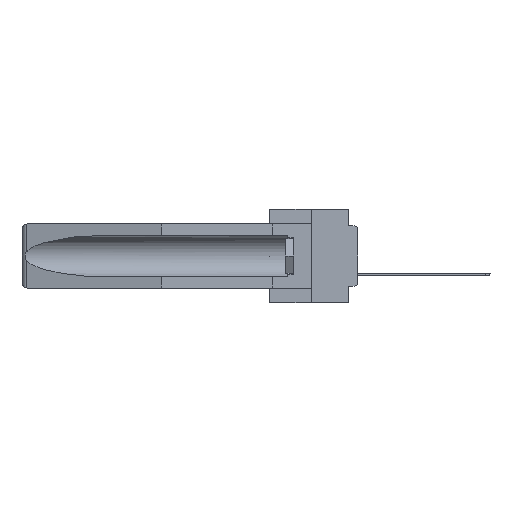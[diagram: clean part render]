
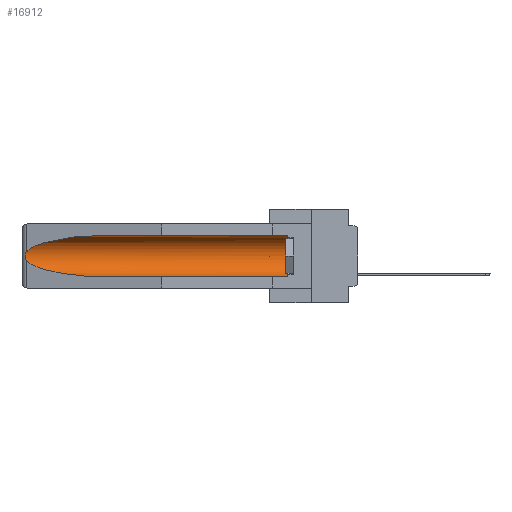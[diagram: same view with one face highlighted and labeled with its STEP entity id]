
A CAD part, left-side view. The second image highlights one B-rep face of the part: STEP entity #16912.
In plain terms, the highlighted cylindrical face has radius 2.857 mm (diameter 5.715 mm), a partial arc.
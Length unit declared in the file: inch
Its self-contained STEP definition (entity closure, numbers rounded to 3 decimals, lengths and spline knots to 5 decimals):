
#337 = ORIENTED_EDGE ( 'NONE', *, *, #30205, .T. ) ;
#547 = FACE_OUTER_BOUND ( 'NONE', #31885, .T. ) ;
#1500 = CARTESIAN_POINT ( 'NONE',  ( 0.155, 0.126, -0.059 ) ) ;
#3882 = CARTESIAN_POINT ( 'NONE',  ( 0.26654, 1.53092, -0.15636 ) ) ;
#4291 = DIRECTION ( 'NONE',  ( 0., 1., 0. ) ) ;
#4937 = CARTESIAN_POINT ( 'NONE',  ( 0.155, -0.30754, -0.284 ) ) ;
#4938 = CARTESIAN_POINT ( 'NONE',  ( 0.155, 0.126, -0.1715 ) ) ;
#5771 = ORIENTED_EDGE ( 'NONE', *, *, #23703, .T. ) ;
#5797 = CARTESIAN_POINT ( 'NONE',  ( 0.21114, 1.30732, -0.059 ) ) ;
#6588 = CARTESIAN_POINT ( 'NONE',  ( 0.2675, 1.53308, -0.16763 ) ) ;
#8005 = VECTOR ( 'NONE', #28163, 39.37008 ) ;
#9463 = CARTESIAN_POINT ( 'NONE',  ( 0.2673, 1.5327, -0.16383 ) ) ;
#11880 = VERTEX_POINT ( 'NONE', #34142 ) ;
#12299 = CARTESIAN_POINT ( 'NONE',  ( 0.26537, 1.52718, -0.19328 ) ) ;
#12626 = LINE ( 'NONE', #4937, #8005 ) ;
#13645 = EDGE_CURVE ( 'NONE', #19716, #15013, #28660, .T. ) ;
#15013 = VERTEX_POINT ( 'NONE', #1500 ) ;
#15052 = ORIENTED_EDGE ( 'NONE', *, *, #20947, .F. ) ;
#15313 = CARTESIAN_POINT ( 'NONE',  ( 0.26597, 1.52961, -0.15275 ) ) ;
#15437 = CARTESIAN_POINT ( 'NONE',  ( 0.26537, 1.52718, -0.14972 ) ) ;
#15881 = CARTESIAN_POINT ( 'NONE',  ( 0.155, 1.07973, -0.059 ) ) ;
#16110 = CARTESIAN_POINT ( 'NONE',  ( 0.155, 0.126, -0.284 ) ) ;
#16495 = EDGE_CURVE ( 'NONE', #33585, #11880, #25370, .T. ) ;
#16912 = ADVANCED_FACE ( 'NONE', ( #547 ), #29380, .F. ) ;
#17400 = AXIS2_PLACEMENT_3D ( 'NONE', #4938, #25728, #37109 ) ;
#18661 = VERTEX_POINT ( 'NONE', #15881 ) ;
#18702 = CARTESIAN_POINT ( 'NONE',  ( 0.2673, 1.53269, -0.17917 ) ) ;
#19716 = VERTEX_POINT ( 'NONE', #16110 ) ;
#19868 = VECTOR ( 'NONE', #36166, 39.37008 ) ;
#20947 = EDGE_CURVE ( 'NONE', #19716, #23461, #12626, .T. ) ;
#22283 = CARTESIAN_POINT ( 'NONE',  ( 0.26537, 1.52718, -0.19328 ) ) ;
#22525 =( BOUNDED_CURVE ( )  B_SPLINE_CURVE ( 3, ( #34262, #5797, #32689, #24079 ),
 .UNSPECIFIED., .F., .F. ) 
 B_SPLINE_CURVE_WITH_KNOTS ( ( 4, 4 ),
 ( 4.71239, 6.08839 ),
 .UNSPECIFIED. ) 
 CURVE ( )  GEOMETRIC_REPRESENTATION_ITEM ( )  RATIONAL_B_SPLINE_CURVE ( ( 1., 0.848, 0.848, 1. ) ) 
 REPRESENTATION_ITEM ( '' )  );
#23461 = VERTEX_POINT ( 'NONE', #33996 ) ;
#23484 = ORIENTED_EDGE ( 'NONE', *, *, #23903, .T. ) ;
#23703 = EDGE_CURVE ( 'NONE', #11880, #23461, #29368, .T. ) ;
#23903 = EDGE_CURVE ( 'NONE', #15013, #18661, #27678, .T. ) ;
#24079 = CARTESIAN_POINT ( 'NONE',  ( 0.26537, 1.52718, -0.14972 ) ) ;
#24775 = CARTESIAN_POINT ( 'NONE',  ( 0.155, -0.30754, -0.059 ) ) ;
#24996 = CARTESIAN_POINT ( 'NONE',  ( 0.155, 1.07973, -0.284 ) ) ;
#25285 = CARTESIAN_POINT ( 'NONE',  ( 0.25451, 1.48313, -0.24835 ) ) ;
#25370 = B_SPLINE_CURVE_WITH_KNOTS ( 'NONE', 3,
 ( #15437, #15313, #3882, #9463, #6588, #30485, #18702, #33081, #36181, #12299 ),
 .UNSPECIFIED., .F., .F.,
 ( 4, 2, 2, 2, 4 ),
 ( 0., 0.00029, 0.00058, 0.00087, 0.00117 ),
 .UNSPECIFIED. ) ;
#25728 = DIRECTION ( 'NONE',  ( 0., -1., 0. ) ) ;
#26277 = ORIENTED_EDGE ( 'NONE', *, *, #16495, .T. ) ;
#27678 = LINE ( 'NONE', #24775, #19868 ) ;
#27808 = CARTESIAN_POINT ( 'NONE',  ( 0.26537, 1.52718, -0.14972 ) ) ;
#27814 = ORIENTED_EDGE ( 'NONE', *, *, #13645, .T. ) ;
#28163 = DIRECTION ( 'NONE',  ( 0., 1., 0. ) ) ;
#28347 = CARTESIAN_POINT ( 'NONE',  ( 0.155, -0.30754, -0.1715 ) ) ;
#28660 = CIRCLE ( 'NONE', #17400, 0.1125 ) ;
#29368 =( BOUNDED_CURVE ( )  B_SPLINE_CURVE ( 3, ( #22283, #25285, #30836, #24996 ),
 .UNSPECIFIED., .F., .F. ) 
 B_SPLINE_CURVE_WITH_KNOTS ( ( 4, 4 ),
 ( 0.1948, 1.5708 ),
 .UNSPECIFIED. ) 
 CURVE ( )  GEOMETRIC_REPRESENTATION_ITEM ( )  RATIONAL_B_SPLINE_CURVE ( ( 1., 0.848, 0.848, 1. ) ) 
 REPRESENTATION_ITEM ( '' )  );
#29380 = CYLINDRICAL_SURFACE ( 'NONE', #37099, 0.1125 ) ;
#30205 = EDGE_CURVE ( 'NONE', #18661, #33585, #22525, .T. ) ;
#30485 = CARTESIAN_POINT ( 'NONE',  ( 0.2675, 1.53308, -0.17534 ) ) ;
#30836 = CARTESIAN_POINT ( 'NONE',  ( 0.21114, 1.30732, -0.284 ) ) ;
#31042 = DIRECTION ( 'NONE',  ( 0., 0., 1. ) ) ;
#31885 = EDGE_LOOP ( 'NONE', ( #337, #26277, #5771, #15052, #27814, #23484 ) ) ;
#32689 = CARTESIAN_POINT ( 'NONE',  ( 0.25451, 1.48313, -0.09465 ) ) ;
#33081 = CARTESIAN_POINT ( 'NONE',  ( 0.26655, 1.53094, -0.18657 ) ) ;
#33585 = VERTEX_POINT ( 'NONE', #27808 ) ;
#33996 = CARTESIAN_POINT ( 'NONE',  ( 0.155, 1.07973, -0.284 ) ) ;
#34142 = CARTESIAN_POINT ( 'NONE',  ( 0.26537, 1.52718, -0.19328 ) ) ;
#34262 = CARTESIAN_POINT ( 'NONE',  ( 0.155, 1.07973, -0.059 ) ) ;
#36166 = DIRECTION ( 'NONE',  ( 0., 1., 0. ) ) ;
#36181 = CARTESIAN_POINT ( 'NONE',  ( 0.26597, 1.5296, -0.19026 ) ) ;
#37099 = AXIS2_PLACEMENT_3D ( 'NONE', #28347, #4291, #31042 ) ;
#37109 = DIRECTION ( 'NONE',  ( 0., 0., 1. ) ) ;
